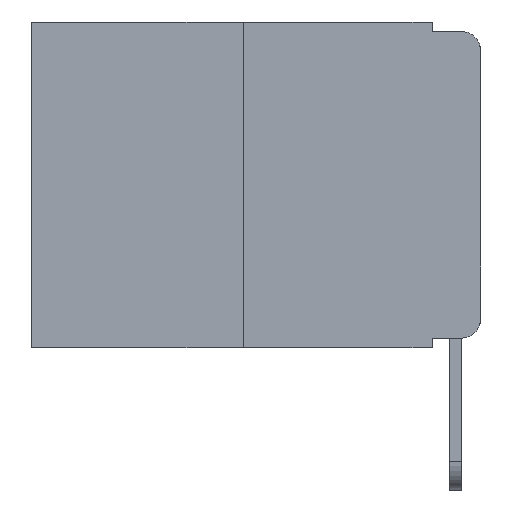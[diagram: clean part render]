
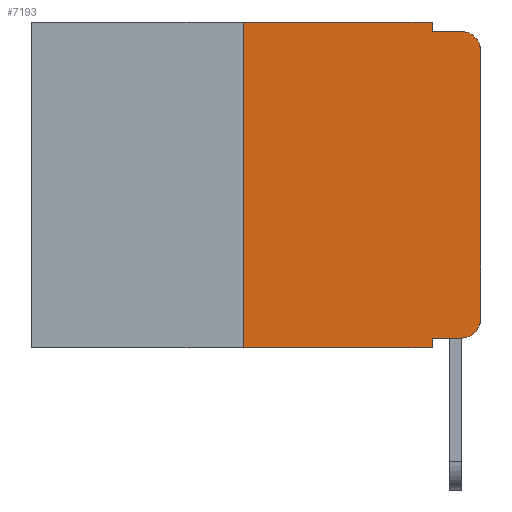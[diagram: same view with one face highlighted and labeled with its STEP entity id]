
A CAD part, left-side view. The second image highlights one B-rep face of the part: STEP entity #7193.
In plain terms, the highlighted planar face has unit normal (-1, 0, 0).
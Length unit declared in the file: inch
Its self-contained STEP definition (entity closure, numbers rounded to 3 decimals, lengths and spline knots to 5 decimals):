
#14 = CARTESIAN_POINT ( 'NONE',  ( 0., 0.02, -0.313 ) ) ;
#146 = CARTESIAN_POINT ( 'NONE',  ( 0., 0.473, 0. ) ) ;
#233 = CARTESIAN_POINT ( 'NONE',  ( 0., 0.02, -0.03 ) ) ;
#666 = CARTESIAN_POINT ( 'NONE',  ( 0., 0.051, -0.343 ) ) ;
#756 = LINE ( 'NONE', #7809, #3044 ) ;
#1088 = VERTEX_POINT ( 'NONE', #3849 ) ;
#1206 = VERTEX_POINT ( 'NONE', #3033 ) ;
#1396 = VECTOR ( 'NONE', #6315, 39.37008 ) ;
#1496 = CARTESIAN_POINT ( 'NONE',  ( 0., 0.25, -0.343 ) ) ;
#1553 = AXIS2_PLACEMENT_3D ( 'NONE', #233, #9902, #9884 ) ;
#1602 = DIRECTION ( 'NONE',  ( 0., 0., 1. ) ) ;
#1713 = VERTEX_POINT ( 'NONE', #2192 ) ;
#1735 = CARTESIAN_POINT ( 'NONE',  ( 0., 0.25, 0. ) ) ;
#2192 = CARTESIAN_POINT ( 'NONE',  ( 0., 0., -0.03 ) ) ;
#2300 = VECTOR ( 'NONE', #3880, 39.37008 ) ;
#2440 = LINE ( 'NONE', #10421, #10831 ) ;
#2526 = ORIENTED_EDGE ( 'NONE', *, *, #2974, .T. ) ;
#2531 = CARTESIAN_POINT ( 'NONE',  ( 0., 0.051, -0.333 ) ) ;
#2806 = DIRECTION ( 'NONE',  ( 0., -1., 0. ) ) ;
#2820 = VERTEX_POINT ( 'NONE', #666 ) ;
#2844 = ORIENTED_EDGE ( 'NONE', *, *, #3042, .F. ) ;
#2897 = EDGE_CURVE ( 'NONE', #3210, #1713, #2440, .T. ) ;
#2974 = EDGE_CURVE ( 'NONE', #1713, #1206, #4024, .T. ) ;
#3033 = CARTESIAN_POINT ( 'NONE',  ( 0., 0.02, -0.01 ) ) ;
#3042 = EDGE_CURVE ( 'NONE', #1088, #1206, #7640, .T. ) ;
#3044 = VECTOR ( 'NONE', #7538, 39.37008 ) ;
#3061 = EDGE_CURVE ( 'NONE', #9559, #1088, #10939, .T. ) ;
#3115 = EDGE_CURVE ( 'NONE', #5943, #9003, #6851, .T. ) ;
#3135 = EDGE_CURVE ( 'NONE', #8405, #2820, #8266, .T. ) ;
#3201 = EDGE_CURVE ( 'NONE', #8405, #6293, #756, .T. ) ;
#3210 = VERTEX_POINT ( 'NONE', #8912 ) ;
#3268 = EDGE_CURVE ( 'NONE', #6293, #3210, #4847, .T. ) ;
#3298 = CARTESIAN_POINT ( 'NONE',  ( 0., 0.051, 0. ) ) ;
#3316 = DIRECTION ( 'NONE',  ( 1., 0., 0. ) ) ;
#3488 = EDGE_LOOP ( 'NONE', ( #6226, #2526, #2844, #4528, #6671, #4796, #6955, #7222, #5356, #7464 ) ) ;
#3849 = CARTESIAN_POINT ( 'NONE',  ( 0., 0.051, -0.01 ) ) ;
#3880 = DIRECTION ( 'NONE',  ( 0., 0., -1. ) ) ;
#3982 = CARTESIAN_POINT ( 'NONE',  ( 0., 0.473, -0.343 ) ) ;
#4024 = CIRCLE ( 'NONE', #1553, 0.02 ) ;
#4059 = EDGE_CURVE ( 'NONE', #9003, #9559, #4322, .T. ) ;
#4322 = LINE ( 'NONE', #146, #8395 ) ;
#4415 = CARTESIAN_POINT ( 'NONE',  ( 0., 0.051, 0. ) ) ;
#4475 = LINE ( 'NONE', #3982, #8521 ) ;
#4528 = ORIENTED_EDGE ( 'NONE', *, *, #3061, .F. ) ;
#4796 = ORIENTED_EDGE ( 'NONE', *, *, #3115, .F. ) ;
#4847 = CIRCLE ( 'NONE', #10180, 0.02 ) ;
#5356 = ORIENTED_EDGE ( 'NONE', *, *, #3201, .T. ) ;
#5943 = VERTEX_POINT ( 'NONE', #1496 ) ;
#6226 = ORIENTED_EDGE ( 'NONE', *, *, #2897, .T. ) ;
#6293 = VERTEX_POINT ( 'NONE', #9601 ) ;
#6294 = DIRECTION ( 'NONE',  ( 0., -1., 0. ) ) ;
#6315 = DIRECTION ( 'NONE',  ( 0., 0., -1. ) ) ;
#6369 = CARTESIAN_POINT ( 'NONE',  ( 0., 0.051, -0.01 ) ) ;
#6671 = ORIENTED_EDGE ( 'NONE', *, *, #4059, .F. ) ;
#6805 = DIRECTION ( 'NONE',  ( 0., 0., 1. ) ) ;
#6851 = LINE ( 'NONE', #10866, #10464 ) ;
#6955 = ORIENTED_EDGE ( 'NONE', *, *, #10107, .T. ) ;
#7149 = VECTOR ( 'NONE', #6294, 39.37008 ) ;
#7193 = ADVANCED_FACE ( 'NONE', ( #9801 ), #10942, .F. ) ;
#7222 = ORIENTED_EDGE ( 'NONE', *, *, #3135, .F. ) ;
#7464 = ORIENTED_EDGE ( 'NONE', *, *, #3268, .T. ) ;
#7491 = CARTESIAN_POINT ( 'NONE',  ( 0., 0.051, 0. ) ) ;
#7538 = DIRECTION ( 'NONE',  ( 0., -1., 0. ) ) ;
#7640 = LINE ( 'NONE', #6369, #7149 ) ;
#7809 = CARTESIAN_POINT ( 'NONE',  ( 0., 0.051, -0.333 ) ) ;
#8241 = DIRECTION ( 'NONE',  ( 0., 0., -1. ) ) ;
#8266 = LINE ( 'NONE', #7491, #1396 ) ;
#8395 = VECTOR ( 'NONE', #2806, 39.37008 ) ;
#8405 = VERTEX_POINT ( 'NONE', #2531 ) ;
#8521 = VECTOR ( 'NONE', #9586, 39.37008 ) ;
#8912 = CARTESIAN_POINT ( 'NONE',  ( 0., 0., -0.313 ) ) ;
#9003 = VERTEX_POINT ( 'NONE', #1735 ) ;
#9301 = DIRECTION ( 'NONE',  ( -1., 0., 0. ) ) ;
#9302 = DIRECTION ( 'NONE',  ( 0., 0., -1. ) ) ;
#9559 = VERTEX_POINT ( 'NONE', #3298 ) ;
#9586 = DIRECTION ( 'NONE',  ( 0., -1., 0. ) ) ;
#9601 = CARTESIAN_POINT ( 'NONE',  ( 0., 0.02, -0.333 ) ) ;
#9801 = FACE_OUTER_BOUND ( 'NONE', #3488, .T. ) ;
#9864 = CARTESIAN_POINT ( 'NONE',  ( 0., 0.473, 0. ) ) ;
#9884 = DIRECTION ( 'NONE',  ( 0., 0., -1. ) ) ;
#9902 = DIRECTION ( 'NONE',  ( -1., 0., 0. ) ) ;
#9921 = AXIS2_PLACEMENT_3D ( 'NONE', #9864, #3316, #8241 ) ;
#10107 = EDGE_CURVE ( 'NONE', #5943, #2820, #4475, .T. ) ;
#10180 = AXIS2_PLACEMENT_3D ( 'NONE', #14, #9301, #9302 ) ;
#10421 = CARTESIAN_POINT ( 'NONE',  ( 0., 0., 0. ) ) ;
#10464 = VECTOR ( 'NONE', #1602, 39.37008 ) ;
#10831 = VECTOR ( 'NONE', #6805, 39.37008 ) ;
#10866 = CARTESIAN_POINT ( 'NONE',  ( 0., 0.25, 0. ) ) ;
#10939 = LINE ( 'NONE', #4415, #2300 ) ;
#10942 = PLANE ( 'NONE',  #9921 ) ;
